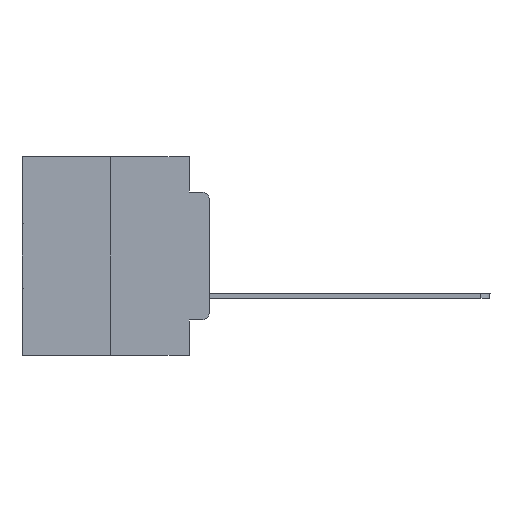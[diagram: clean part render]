
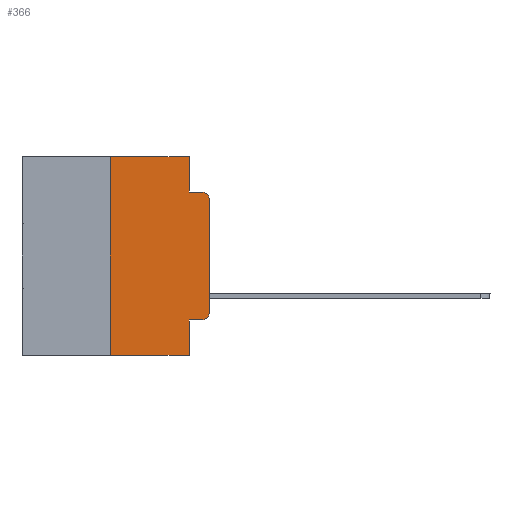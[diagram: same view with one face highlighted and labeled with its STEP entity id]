
A CAD part, left-side view. The second image highlights one B-rep face of the part: STEP entity #366.
In plain terms, the highlighted planar face has unit normal (-1, 0, 0).
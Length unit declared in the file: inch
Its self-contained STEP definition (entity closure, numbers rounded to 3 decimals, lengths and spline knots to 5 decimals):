
#258 = DIRECTION ( 'NONE',  ( 0., 0., -1. ) ) ;
#366 = ADVANCED_FACE ( 'NONE', ( #27397 ), #11253, .F. ) ;
#1158 = DIRECTION ( 'NONE',  ( 0., -1., 0. ) ) ;
#2777 = ORIENTED_EDGE ( 'NONE', *, *, #29934, .F. ) ;
#3094 = DIRECTION ( 'NONE',  ( 0., 0., -1. ) ) ;
#3327 = CARTESIAN_POINT ( 'NONE',  ( 0., 0.051, 0. ) ) ;
#3420 = DIRECTION ( 'NONE',  ( 0., 0., -1. ) ) ;
#3516 = VECTOR ( 'NONE', #20956, 39.37008 ) ;
#3772 = AXIS2_PLACEMENT_3D ( 'NONE', #8832, #5028, #7630 ) ;
#4016 = VERTEX_POINT ( 'NONE', #26963 ) ;
#4189 = DIRECTION ( 'NONE',  ( 0., 0., -1. ) ) ;
#5028 = DIRECTION ( 'NONE',  ( 1., 0., 0. ) ) ;
#5234 = VERTEX_POINT ( 'NONE', #6430 ) ;
#6430 = CARTESIAN_POINT ( 'NONE',  ( 0., 0.051, -0.0885 ) ) ;
#7085 = CIRCLE ( 'NONE', #21123, 0.02 ) ;
#7369 = CARTESIAN_POINT ( 'NONE',  ( 0., 0., -0.1085 ) ) ;
#7630 = DIRECTION ( 'NONE',  ( 0., 0., -1. ) ) ;
#7716 = DIRECTION ( 'NONE',  ( -1., 0., 0. ) ) ;
#8832 = CARTESIAN_POINT ( 'NONE',  ( 0., 0.473, 0. ) ) ;
#8931 = CARTESIAN_POINT ( 'NONE',  ( 0., 0.051, -0.4115 ) ) ;
#9096 = DIRECTION ( 'NONE',  ( 0., -1., 0. ) ) ;
#9995 = VECTOR ( 'NONE', #4189, 39.37008 ) ;
#10729 = CARTESIAN_POINT ( 'NONE',  ( 0., 0.051, 0. ) ) ;
#10942 = CIRCLE ( 'NONE', #24531, 0.02 ) ;
#11221 = LINE ( 'NONE', #27815, #18609 ) ;
#11253 = PLANE ( 'NONE',  #3772 ) ;
#11731 = VERTEX_POINT ( 'NONE', #13536 ) ;
#12442 = EDGE_CURVE ( 'NONE', #23606, #11731, #22135, .T. ) ;
#13346 = EDGE_CURVE ( 'NONE', #25651, #23040, #15187, .T. ) ;
#13435 = ORIENTED_EDGE ( 'NONE', *, *, #14223, .F. ) ;
#13536 = CARTESIAN_POINT ( 'NONE',  ( 0., 0.051, -0.5 ) ) ;
#13700 = CARTESIAN_POINT ( 'NONE',  ( 0., 0.25, -0.5 ) ) ;
#14047 = ORIENTED_EDGE ( 'NONE', *, *, #12442, .T. ) ;
#14223 = EDGE_CURVE ( 'NONE', #25651, #11731, #11221, .T. ) ;
#14264 = LINE ( 'NONE', #14418, #18690 ) ;
#14418 = CARTESIAN_POINT ( 'NONE',  ( 0., 0.473, 0. ) ) ;
#14742 = VECTOR ( 'NONE', #27824, 39.37008 ) ;
#15187 = LINE ( 'NONE', #22179, #3516 ) ;
#16416 = EDGE_CURVE ( 'NONE', #22089, #24536, #7085, .T. ) ;
#17119 = ORIENTED_EDGE ( 'NONE', *, *, #16416, .T. ) ;
#17168 = ORIENTED_EDGE ( 'NONE', *, *, #28489, .T. ) ;
#17265 = CARTESIAN_POINT ( 'NONE',  ( 0., 0.02, -0.4115 ) ) ;
#18531 = CARTESIAN_POINT ( 'NONE',  ( 0., 0., 0. ) ) ;
#18609 = VECTOR ( 'NONE', #258, 39.37008 ) ;
#18690 = VECTOR ( 'NONE', #19146, 39.37008 ) ;
#19146 = DIRECTION ( 'NONE',  ( 0., -1., 0. ) ) ;
#19216 = CARTESIAN_POINT ( 'NONE',  ( 0., 0.02, -0.1085 ) ) ;
#19465 = CARTESIAN_POINT ( 'NONE',  ( 0., 0., -0.3915 ) ) ;
#19980 = DIRECTION ( 'NONE',  ( 0., 0., 1. ) ) ;
#19992 = VERTEX_POINT ( 'NONE', #10729 ) ;
#20019 = CARTESIAN_POINT ( 'NONE',  ( 0., 0.473, -0.5 ) ) ;
#20874 = ORIENTED_EDGE ( 'NONE', *, *, #13346, .T. ) ;
#20956 = DIRECTION ( 'NONE',  ( 0., -1., 0. ) ) ;
#21123 = AXIS2_PLACEMENT_3D ( 'NONE', #19216, #28520, #3094 ) ;
#21278 = VERTEX_POINT ( 'NONE', #19465 ) ;
#21334 = ORIENTED_EDGE ( 'NONE', *, *, #26631, .T. ) ;
#21636 = EDGE_CURVE ( 'NONE', #5234, #24536, #25979, .T. ) ;
#21736 = EDGE_CURVE ( 'NONE', #23606, #4016, #28838, .T. ) ;
#22089 = VERTEX_POINT ( 'NONE', #7369 ) ;
#22135 = LINE ( 'NONE', #20019, #24902 ) ;
#22179 = CARTESIAN_POINT ( 'NONE',  ( 0., 0.051, -0.4115 ) ) ;
#22284 = VECTOR ( 'NONE', #9096, 39.37008 ) ;
#22649 = ORIENTED_EDGE ( 'NONE', *, *, #21636, .F. ) ;
#23040 = VERTEX_POINT ( 'NONE', #17265 ) ;
#23606 = VERTEX_POINT ( 'NONE', #13700 ) ;
#24254 = CARTESIAN_POINT ( 'NONE',  ( 0., 0.02, -0.3915 ) ) ;
#24531 = AXIS2_PLACEMENT_3D ( 'NONE', #24254, #7716, #3420 ) ;
#24536 = VERTEX_POINT ( 'NONE', #27127 ) ;
#24604 = ORIENTED_EDGE ( 'NONE', *, *, #27886, .F. ) ;
#24860 = LINE ( 'NONE', #3327, #9995 ) ;
#24902 = VECTOR ( 'NONE', #1158, 39.37008 ) ;
#25651 = VERTEX_POINT ( 'NONE', #8931 ) ;
#25819 = CARTESIAN_POINT ( 'NONE',  ( 0., 0.051, -0.0885 ) ) ;
#25979 = LINE ( 'NONE', #25819, #22284 ) ;
#26631 = EDGE_CURVE ( 'NONE', #21278, #22089, #30115, .T. ) ;
#26671 = VECTOR ( 'NONE', #19980, 39.37008 ) ;
#26963 = CARTESIAN_POINT ( 'NONE',  ( 0., 0.25, 0. ) ) ;
#27127 = CARTESIAN_POINT ( 'NONE',  ( 0., 0.02, -0.0885 ) ) ;
#27397 = FACE_OUTER_BOUND ( 'NONE', #28858, .T. ) ;
#27513 = ORIENTED_EDGE ( 'NONE', *, *, #21736, .F. ) ;
#27815 = CARTESIAN_POINT ( 'NONE',  ( 0., 0.051, 0. ) ) ;
#27824 = DIRECTION ( 'NONE',  ( 0., 0., 1. ) ) ;
#27886 = EDGE_CURVE ( 'NONE', #4016, #19992, #14264, .T. ) ;
#28489 = EDGE_CURVE ( 'NONE', #23040, #21278, #10942, .T. ) ;
#28520 = DIRECTION ( 'NONE',  ( -1., 0., 0. ) ) ;
#28838 = LINE ( 'NONE', #29135, #26671 ) ;
#28858 = EDGE_LOOP ( 'NONE', ( #21334, #17119, #22649, #2777, #24604, #27513, #14047, #13435, #20874, #17168 ) ) ;
#29135 = CARTESIAN_POINT ( 'NONE',  ( 0., 0.25, 0. ) ) ;
#29934 = EDGE_CURVE ( 'NONE', #19992, #5234, #24860, .T. ) ;
#30115 = LINE ( 'NONE', #18531, #14742 ) ;
